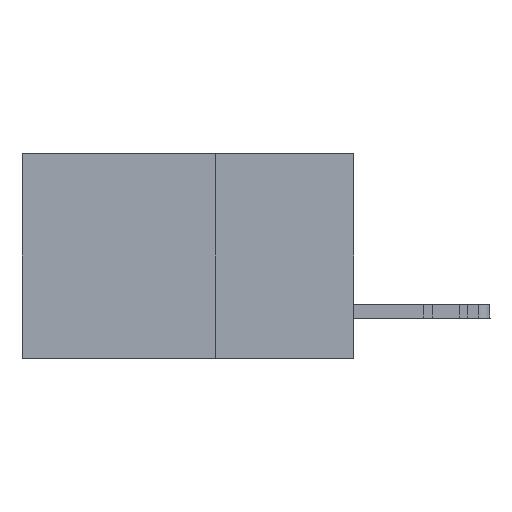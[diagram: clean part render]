
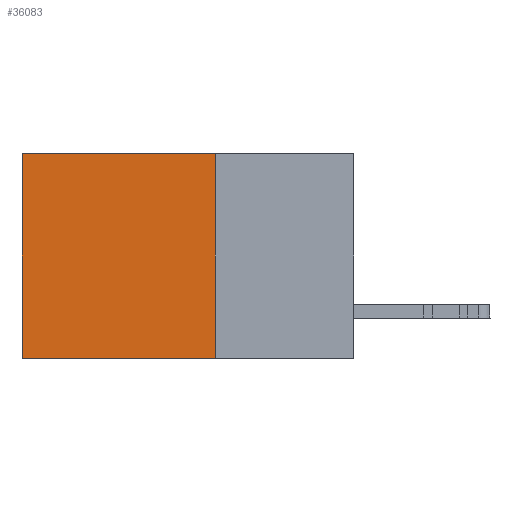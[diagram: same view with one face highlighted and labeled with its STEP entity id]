
A CAD part, left-side view. The second image highlights one B-rep face of the part: STEP entity #36083.
In plain terms, the highlighted planar face has unit normal (-1, 0, 0).
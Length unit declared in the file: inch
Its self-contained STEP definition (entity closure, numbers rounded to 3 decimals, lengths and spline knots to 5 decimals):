
#1438 = CARTESIAN_POINT ( 'NONE',  ( 0.2875, 0.6, -0.37 ) ) ;
#2861 = VERTEX_POINT ( 'NONE', #34190 ) ;
#7268 = ORIENTED_EDGE ( 'NONE', *, *, #18089, .F. ) ;
#7579 = DIRECTION ( 'NONE',  ( 0., 0., -1. ) ) ;
#7651 = CARTESIAN_POINT ( 'NONE',  ( 0.2875, 0.6, 0. ) ) ;
#7847 = VECTOR ( 'NONE', #37446, 39.37008 ) ;
#9624 = DIRECTION ( 'NONE',  ( 0., 1., 0. ) ) ;
#10112 = EDGE_LOOP ( 'NONE', ( #33403, #7268, #41375, #11378 ) ) ;
#11143 = AXIS2_PLACEMENT_3D ( 'NONE', #14761, #31723, #34805 ) ;
#11378 = ORIENTED_EDGE ( 'NONE', *, *, #42196, .T. ) ;
#12538 = VECTOR ( 'NONE', #7579, 39.37008 ) ;
#12977 = CARTESIAN_POINT ( 'NONE',  ( 0.2875, 0.25, -0.37 ) ) ;
#14544 = DIRECTION ( 'NONE',  ( 0., 0., -1. ) ) ;
#14761 = CARTESIAN_POINT ( 'NONE',  ( 0.2875, 0.25, 0. ) ) ;
#14976 = VERTEX_POINT ( 'NONE', #28726 ) ;
#16335 = VERTEX_POINT ( 'NONE', #1438 ) ;
#18089 = EDGE_CURVE ( 'NONE', #41137, #16335, #24591, .T. ) ;
#20848 = VECTOR ( 'NONE', #9624, 39.37008 ) ;
#21648 = PLANE ( 'NONE',  #11143 ) ;
#23677 = EDGE_CURVE ( 'NONE', #14976, #16335, #29589, .T. ) ;
#24115 = FACE_OUTER_BOUND ( 'NONE', #10112, .T. ) ;
#24591 = LINE ( 'NONE', #30761, #7847 ) ;
#25939 = VECTOR ( 'NONE', #14544, 39.37008 ) ;
#28726 = CARTESIAN_POINT ( 'NONE',  ( 0.2875, 0.6, 0. ) ) ;
#29589 = LINE ( 'NONE', #7651, #25939 ) ;
#29845 = EDGE_CURVE ( 'NONE', #2861, #41137, #34827, .T. ) ;
#30761 = CARTESIAN_POINT ( 'NONE',  ( 0.2875, 0.25, -0.37 ) ) ;
#31723 = DIRECTION ( 'NONE',  ( 1., 0., 0. ) ) ;
#33403 = ORIENTED_EDGE ( 'NONE', *, *, #23677, .T. ) ;
#34190 = CARTESIAN_POINT ( 'NONE',  ( 0.2875, 0.25, 0. ) ) ;
#34805 = DIRECTION ( 'NONE',  ( 0., 0., -1. ) ) ;
#34827 = LINE ( 'NONE', #41044, #12538 ) ;
#36083 = ADVANCED_FACE ( 'NONE', ( #24115 ), #21648, .F. ) ;
#36097 = LINE ( 'NONE', #39826, #20848 ) ;
#37446 = DIRECTION ( 'NONE',  ( 0., 1., 0. ) ) ;
#39826 = CARTESIAN_POINT ( 'NONE',  ( 0.2875, 0.25, 0. ) ) ;
#41044 = CARTESIAN_POINT ( 'NONE',  ( 0.2875, 0.25, 0. ) ) ;
#41137 = VERTEX_POINT ( 'NONE', #12977 ) ;
#41375 = ORIENTED_EDGE ( 'NONE', *, *, #29845, .F. ) ;
#42196 = EDGE_CURVE ( 'NONE', #2861, #14976, #36097, .T. ) ;
